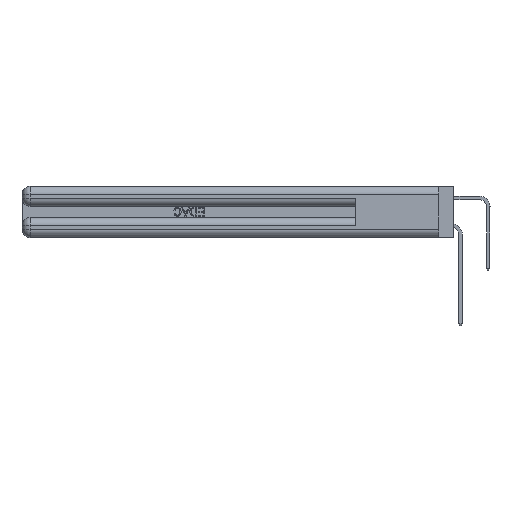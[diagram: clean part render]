
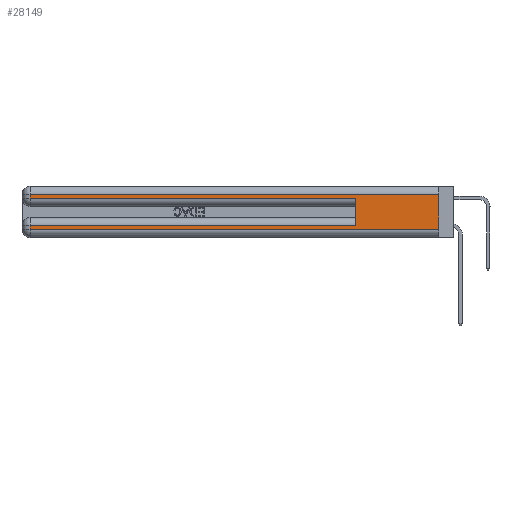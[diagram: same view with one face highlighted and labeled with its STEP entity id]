
A CAD part, left-side view. The second image highlights one B-rep face of the part: STEP entity #28149.
In plain terms, the highlighted planar face has unit normal (-1, 0, 0).
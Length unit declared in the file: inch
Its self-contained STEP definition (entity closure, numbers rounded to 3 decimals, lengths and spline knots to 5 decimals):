
#209 = LINE ( 'NONE', #4511, #8416 ) ;
#255 = DIRECTION ( 'NONE',  ( 0., 0., -1. ) ) ;
#458 = VECTOR ( 'NONE', #12229, 39.37008 ) ;
#879 = CARTESIAN_POINT ( 'NONE',  ( 0., 0., 0.31 ) ) ;
#1513 = EDGE_LOOP ( 'NONE', ( #26704, #27518, #12039, #7904, #14765, #33981, #13146, #3038 ) ) ;
#1580 = FACE_OUTER_BOUND ( 'NONE', #1513, .T. ) ;
#2387 = CARTESIAN_POINT ( 'NONE',  ( 0., 0.6, 0.145 ) ) ;
#3038 = ORIENTED_EDGE ( 'NONE', *, *, #32367, .T. ) ;
#3779 = VERTEX_POINT ( 'NONE', #29157 ) ;
#3960 = VECTOR ( 'NONE', #6483, 39.37008 ) ;
#4511 = CARTESIAN_POINT ( 'NONE',  ( 0., 0., 0.37 ) ) ;
#5440 = VERTEX_POINT ( 'NONE', #28510 ) ;
#5896 = VERTEX_POINT ( 'NONE', #11976 ) ;
#6318 = CARTESIAN_POINT ( 'NONE',  ( 0., 2.94, 0.37 ) ) ;
#6483 = DIRECTION ( 'NONE',  ( 0., -1., 0. ) ) ;
#6983 = EDGE_CURVE ( 'NONE', #5440, #19115, #23803, .T. ) ;
#7707 = LINE ( 'NONE', #27593, #458 ) ;
#7904 = ORIENTED_EDGE ( 'NONE', *, *, #15955, .T. ) ;
#8416 = VECTOR ( 'NONE', #28962, 39.37008 ) ;
#9918 = EDGE_CURVE ( 'NONE', #37162, #28613, #20308, .T. ) ;
#10467 = LINE ( 'NONE', #24071, #33696 ) ;
#11976 = CARTESIAN_POINT ( 'NONE',  ( 0., 2.94, 0.085 ) ) ;
#12039 = ORIENTED_EDGE ( 'NONE', *, *, #38309, .T. ) ;
#12225 = VECTOR ( 'NONE', #17507, 39.37008 ) ;
#12229 = DIRECTION ( 'NONE',  ( 0., 0., -1. ) ) ;
#12624 = CARTESIAN_POINT ( 'NONE',  ( 0., 0.6, 0.285 ) ) ;
#13146 = ORIENTED_EDGE ( 'NONE', *, *, #38269, .T. ) ;
#13767 = CARTESIAN_POINT ( 'NONE',  ( 0., 2.94, 0.285 ) ) ;
#13842 = CARTESIAN_POINT ( 'NONE',  ( 0., 0., 0.37 ) ) ;
#14002 = CARTESIAN_POINT ( 'NONE',  ( 0., 2.94, 0.06 ) ) ;
#14765 = ORIENTED_EDGE ( 'NONE', *, *, #6983, .F. ) ;
#15955 = EDGE_CURVE ( 'NONE', #35493, #19115, #10467, .T. ) ;
#16915 = DIRECTION ( 'NONE',  ( 1., 0., 0. ) ) ;
#17378 = CARTESIAN_POINT ( 'NONE',  ( 0., 0., 0.085 ) ) ;
#17507 = DIRECTION ( 'NONE',  ( 0., 1., 0. ) ) ;
#17685 = DIRECTION ( 'NONE',  ( 0., 0., 1. ) ) ;
#18753 = VERTEX_POINT ( 'NONE', #14002 ) ;
#19115 = VERTEX_POINT ( 'NONE', #12624 ) ;
#19194 = CARTESIAN_POINT ( 'NONE',  ( 0., 2.94, 0.31 ) ) ;
#20308 = LINE ( 'NONE', #38661, #27399 ) ;
#20432 = LINE ( 'NONE', #17378, #12225 ) ;
#20880 = DIRECTION ( 'NONE',  ( 0., -1., 0. ) ) ;
#22115 = LINE ( 'NONE', #6318, #37035 ) ;
#23803 = LINE ( 'NONE', #2387, #38693 ) ;
#23920 = AXIS2_PLACEMENT_3D ( 'NONE', #13842, #16915, #37958 ) ;
#24071 = CARTESIAN_POINT ( 'NONE',  ( 0., 0., 0.285 ) ) ;
#26704 = ORIENTED_EDGE ( 'NONE', *, *, #27020, .F. ) ;
#27020 = EDGE_CURVE ( 'NONE', #37162, #3779, #209, .T. ) ;
#27399 = VECTOR ( 'NONE', #29845, 39.37008 ) ;
#27518 = ORIENTED_EDGE ( 'NONE', *, *, #9918, .T. ) ;
#27593 = CARTESIAN_POINT ( 'NONE',  ( 0., 2.94, 0.37 ) ) ;
#27884 = CARTESIAN_POINT ( 'NONE',  ( 0., 0., 0.06 ) ) ;
#28149 = ADVANCED_FACE ( 'NONE', ( #1580 ), #32000, .F. ) ;
#28360 = LINE ( 'NONE', #27884, #3960 ) ;
#28510 = CARTESIAN_POINT ( 'NONE',  ( 0., 0.6, 0.085 ) ) ;
#28613 = VERTEX_POINT ( 'NONE', #19194 ) ;
#28962 = DIRECTION ( 'NONE',  ( 0., 0., -1. ) ) ;
#29157 = CARTESIAN_POINT ( 'NONE',  ( 0., 0., 0.06 ) ) ;
#29845 = DIRECTION ( 'NONE',  ( 0., 1., 0. ) ) ;
#30256 = EDGE_CURVE ( 'NONE', #5440, #5896, #20432, .T. ) ;
#32000 = PLANE ( 'NONE',  #23920 ) ;
#32367 = EDGE_CURVE ( 'NONE', #18753, #3779, #28360, .T. ) ;
#33696 = VECTOR ( 'NONE', #20880, 39.37008 ) ;
#33981 = ORIENTED_EDGE ( 'NONE', *, *, #30256, .T. ) ;
#35493 = VERTEX_POINT ( 'NONE', #13767 ) ;
#37035 = VECTOR ( 'NONE', #255, 39.37008 ) ;
#37162 = VERTEX_POINT ( 'NONE', #879 ) ;
#37958 = DIRECTION ( 'NONE',  ( 0., 0., -1. ) ) ;
#38269 = EDGE_CURVE ( 'NONE', #5896, #18753, #7707, .T. ) ;
#38309 = EDGE_CURVE ( 'NONE', #28613, #35493, #22115, .T. ) ;
#38661 = CARTESIAN_POINT ( 'NONE',  ( 0., 0., 0.31 ) ) ;
#38693 = VECTOR ( 'NONE', #17685, 39.37008 ) ;
